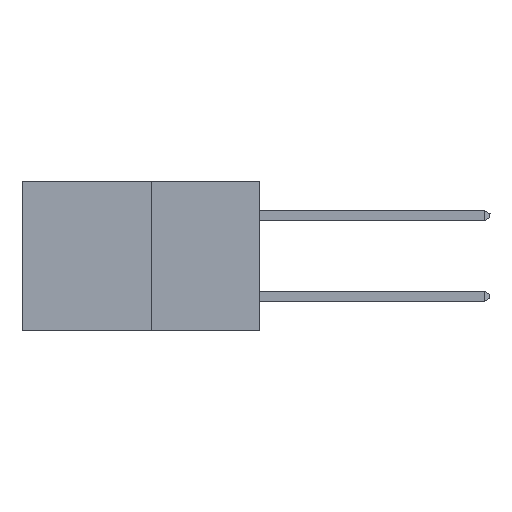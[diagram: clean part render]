
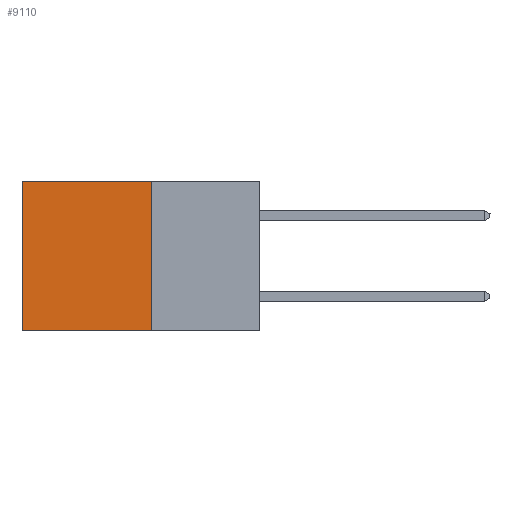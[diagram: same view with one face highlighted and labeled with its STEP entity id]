
A CAD part, left-side view. The second image highlights one B-rep face of the part: STEP entity #9110.
In plain terms, the highlighted planar face has unit normal (-1, 0, 0).
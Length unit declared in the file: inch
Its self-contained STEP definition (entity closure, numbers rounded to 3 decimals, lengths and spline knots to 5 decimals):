
#170 = ORIENTED_EDGE ( 'NONE', *, *, #3314, .F. ) ;
#415 = DIRECTION ( 'NONE',  ( 0., 0., -1. ) ) ;
#419 = DIRECTION ( 'NONE',  ( 1., 0., 0. ) ) ;
#434 = PLANE ( 'NONE',  #1790 ) ;
#463 = CARTESIAN_POINT ( 'NONE',  ( 0.277, 0.27, -0.37 ) ) ;
#616 = EDGE_CURVE ( 'NONE', #5644, #5381, #8618, .T. ) ;
#1059 = CARTESIAN_POINT ( 'NONE',  ( 0.277, 0.27, -0.37 ) ) ;
#1790 = AXIS2_PLACEMENT_3D ( 'NONE', #463, #419, #415 ) ;
#1893 = CARTESIAN_POINT ( 'NONE',  ( 0.277, 0.27, 0. ) ) ;
#2399 = CARTESIAN_POINT ( 'NONE',  ( 0.277, 0.59, 0. ) ) ;
#3050 = DIRECTION ( 'NONE',  ( 0., 1., 0. ) ) ;
#3314 = EDGE_CURVE ( 'NONE', #12601, #8997, #3379, .T. ) ;
#3379 = LINE ( 'NONE', #11069, #5963 ) ;
#3699 = CARTESIAN_POINT ( 'NONE',  ( 0.277, 0.59, -0.37 ) ) ;
#3836 = LINE ( 'NONE', #1893, #9354 ) ;
#4408 = ORIENTED_EDGE ( 'NONE', *, *, #6027, .T. ) ;
#4476 = DIRECTION ( 'NONE',  ( 0., 0., -1. ) ) ;
#4822 = CARTESIAN_POINT ( 'NONE',  ( 0.277, 0.59, -0.37 ) ) ;
#5038 = EDGE_CURVE ( 'NONE', #8997, #5381, #10584, .T. ) ;
#5381 = VERTEX_POINT ( 'NONE', #4822 ) ;
#5644 = VERTEX_POINT ( 'NONE', #2399 ) ;
#5963 = VECTOR ( 'NONE', #10890, 39.37008 ) ;
#6027 = EDGE_CURVE ( 'NONE', #12601, #5644, #3836, .T. ) ;
#8097 = DIRECTION ( 'NONE',  ( 0., 1., 0. ) ) ;
#8111 = CARTESIAN_POINT ( 'NONE',  ( 0.277, 0.27, -0.37 ) ) ;
#8130 = EDGE_LOOP ( 'NONE', ( #9480, #8356, #170, #4408 ) ) ;
#8356 = ORIENTED_EDGE ( 'NONE', *, *, #5038, .F. ) ;
#8618 = LINE ( 'NONE', #3699, #14084 ) ;
#8997 = VERTEX_POINT ( 'NONE', #1059 ) ;
#9110 = ADVANCED_FACE ( 'NONE', ( #13296 ), #434, .F. ) ;
#9354 = VECTOR ( 'NONE', #3050, 39.37008 ) ;
#9480 = ORIENTED_EDGE ( 'NONE', *, *, #616, .T. ) ;
#10584 = LINE ( 'NONE', #8111, #13495 ) ;
#10890 = DIRECTION ( 'NONE',  ( 0., 0., -1. ) ) ;
#11069 = CARTESIAN_POINT ( 'NONE',  ( 0.277, 0.27, -0.37 ) ) ;
#12601 = VERTEX_POINT ( 'NONE', #14109 ) ;
#13296 = FACE_OUTER_BOUND ( 'NONE', #8130, .T. ) ;
#13495 = VECTOR ( 'NONE', #8097, 39.37008 ) ;
#14084 = VECTOR ( 'NONE', #4476, 39.37008 ) ;
#14109 = CARTESIAN_POINT ( 'NONE',  ( 0.277, 0.27, 0. ) ) ;
